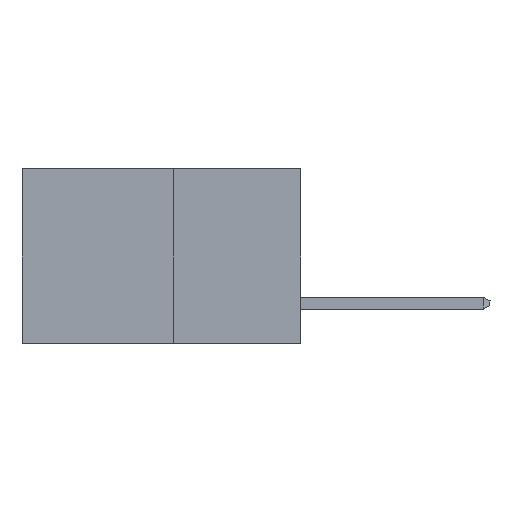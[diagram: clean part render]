
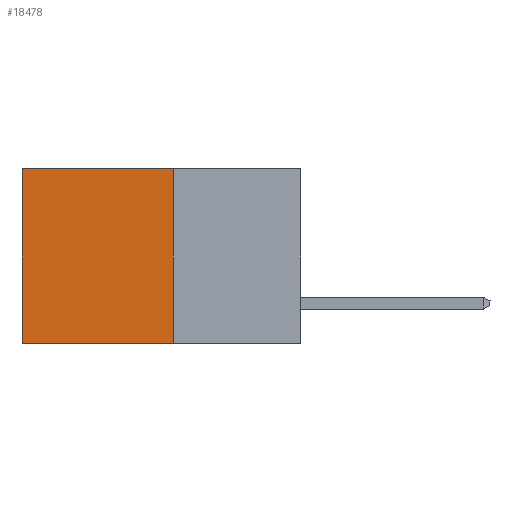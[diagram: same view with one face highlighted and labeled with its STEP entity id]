
A CAD part, left-side view. The second image highlights one B-rep face of the part: STEP entity #18478.
In plain terms, the highlighted planar face has unit normal (-1, 0, 0).
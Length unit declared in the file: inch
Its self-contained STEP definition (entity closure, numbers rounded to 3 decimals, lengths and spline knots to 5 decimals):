
#245 = VERTEX_POINT ( 'NONE', #18347 ) ;
#764 = CARTESIAN_POINT ( 'NONE',  ( 0.277, 0.27, -0.37 ) ) ;
#1267 = DIRECTION ( 'NONE',  ( 0., 1., 0. ) ) ;
#2791 = DIRECTION ( 'NONE',  ( 0., 0., -1. ) ) ;
#2965 = CARTESIAN_POINT ( 'NONE',  ( 0.277, 0.27, -0.37 ) ) ;
#3284 = CARTESIAN_POINT ( 'NONE',  ( 0.277, 0.59, -0.37 ) ) ;
#4868 = VECTOR ( 'NONE', #13221, 39.37008 ) ;
#6977 = DIRECTION ( 'NONE',  ( 1., 0., 0. ) ) ;
#7230 = CARTESIAN_POINT ( 'NONE',  ( 0.277, 0.27, -0.37 ) ) ;
#7244 = DIRECTION ( 'NONE',  ( 0., 1., 0. ) ) ;
#9585 = VECTOR ( 'NONE', #7244, 39.37008 ) ;
#10020 = FACE_OUTER_BOUND ( 'NONE', #19929, .T. ) ;
#11176 = CARTESIAN_POINT ( 'NONE',  ( 0.277, 0.59, -0.37 ) ) ;
#12233 = EDGE_CURVE ( 'NONE', #18379, #17416, #23185, .T. ) ;
#12378 = LINE ( 'NONE', #764, #22533 ) ;
#13221 = DIRECTION ( 'NONE',  ( 0., 0., -1. ) ) ;
#14200 = VERTEX_POINT ( 'NONE', #15614 ) ;
#15153 = AXIS2_PLACEMENT_3D ( 'NONE', #2965, #6977, #21218 ) ;
#15474 = ORIENTED_EDGE ( 'NONE', *, *, #22265, .F. ) ;
#15614 = CARTESIAN_POINT ( 'NONE',  ( 0.277, 0.27, 0. ) ) ;
#15667 = LINE ( 'NONE', #11176, #4868 ) ;
#17416 = VERTEX_POINT ( 'NONE', #3284 ) ;
#17849 = VECTOR ( 'NONE', #1267, 39.37008 ) ;
#18347 = CARTESIAN_POINT ( 'NONE',  ( 0.277, 0.59, 0. ) ) ;
#18379 = VERTEX_POINT ( 'NONE', #20968 ) ;
#18478 = ADVANCED_FACE ( 'NONE', ( #10020 ), #21137, .F. ) ;
#19175 = LINE ( 'NONE', #21480, #9585 ) ;
#19929 = EDGE_LOOP ( 'NONE', ( #24479, #21104, #15474, #22570 ) ) ;
#20443 = EDGE_CURVE ( 'NONE', #245, #17416, #15667, .T. ) ;
#20476 = EDGE_CURVE ( 'NONE', #14200, #245, #19175, .T. ) ;
#20968 = CARTESIAN_POINT ( 'NONE',  ( 0.277, 0.27, -0.37 ) ) ;
#21104 = ORIENTED_EDGE ( 'NONE', *, *, #12233, .F. ) ;
#21137 = PLANE ( 'NONE',  #15153 ) ;
#21218 = DIRECTION ( 'NONE',  ( 0., 0., -1. ) ) ;
#21480 = CARTESIAN_POINT ( 'NONE',  ( 0.277, 0.27, 0. ) ) ;
#22265 = EDGE_CURVE ( 'NONE', #14200, #18379, #12378, .T. ) ;
#22533 = VECTOR ( 'NONE', #2791, 39.37008 ) ;
#22570 = ORIENTED_EDGE ( 'NONE', *, *, #20476, .T. ) ;
#23185 = LINE ( 'NONE', #7230, #17849 ) ;
#24479 = ORIENTED_EDGE ( 'NONE', *, *, #20443, .T. ) ;
